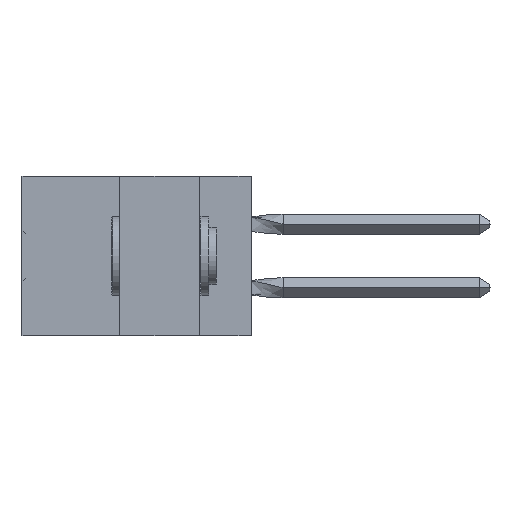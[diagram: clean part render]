
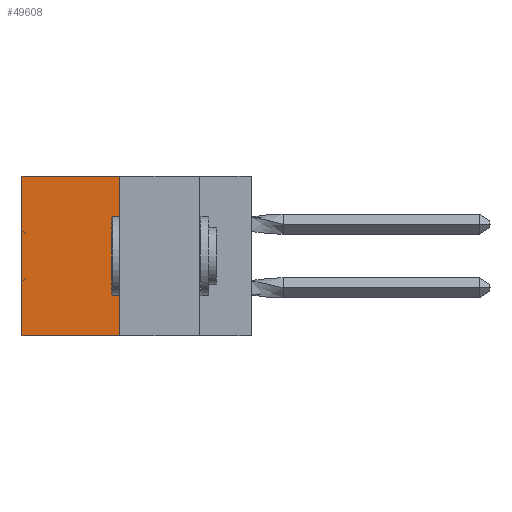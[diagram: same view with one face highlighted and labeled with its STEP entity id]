
A CAD part, left-side view. The second image highlights one B-rep face of the part: STEP entity #49608.
In plain terms, the highlighted planar face has unit normal (-1, 0, 0).
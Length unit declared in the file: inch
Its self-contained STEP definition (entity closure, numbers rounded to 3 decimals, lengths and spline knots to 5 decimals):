
#1169 = FACE_OUTER_BOUND ( 'NONE', #30408, .T. ) ;
#4736 = VECTOR ( 'NONE', #14009, 39.37008 ) ;
#5809 = VECTOR ( 'NONE', #36011, 39.37008 ) ;
#7497 = DIRECTION ( 'NONE',  ( 0., 1., 0. ) ) ;
#10159 = DIRECTION ( 'NONE',  ( 1., 0., 0. ) ) ;
#11826 = VERTEX_POINT ( 'NONE', #25598 ) ;
#12206 = LINE ( 'NONE', #53501, #4736 ) ;
#12739 = ORIENTED_EDGE ( 'NONE', *, *, #55975, .F. ) ;
#13294 = ORIENTED_EDGE ( 'NONE', *, *, #40919, .T. ) ;
#14009 = DIRECTION ( 'NONE',  ( 0., 0., -1. ) ) ;
#16894 = CARTESIAN_POINT ( 'NONE',  ( 0.305, 0.413, -0.5 ) ) ;
#19998 = EDGE_CURVE ( 'NONE', #11826, #40989, #12206, .T. ) ;
#22746 = CARTESIAN_POINT ( 'NONE',  ( 0.305, 0.413, -0.5 ) ) ;
#23274 = EDGE_CURVE ( 'NONE', #36505, #25533, #39822, .T. ) ;
#25533 = VERTEX_POINT ( 'NONE', #16894 ) ;
#25598 = CARTESIAN_POINT ( 'NONE',  ( 0.305, 0.72, 0. ) ) ;
#26746 = DIRECTION ( 'NONE',  ( 0., 1., 0. ) ) ;
#28204 = AXIS2_PLACEMENT_3D ( 'NONE', #22746, #10159, #40622 ) ;
#30408 = EDGE_LOOP ( 'NONE', ( #51049, #12739, #38060, #13294 ) ) ;
#31680 = VECTOR ( 'NONE', #7497, 39.37008 ) ;
#33910 = CARTESIAN_POINT ( 'NONE',  ( 0.305, 0.413, 0. ) ) ;
#34070 = VECTOR ( 'NONE', #26746, 39.37008 ) ;
#36011 = DIRECTION ( 'NONE',  ( 0., 0., -1. ) ) ;
#36232 = PLANE ( 'NONE',  #28204 ) ;
#36505 = VERTEX_POINT ( 'NONE', #37008 ) ;
#37008 = CARTESIAN_POINT ( 'NONE',  ( 0.305, 0.413, 0. ) ) ;
#38060 = ORIENTED_EDGE ( 'NONE', *, *, #23274, .F. ) ;
#39822 = LINE ( 'NONE', #44814, #5809 ) ;
#39830 = LINE ( 'NONE', #33910, #31680 ) ;
#39969 = CARTESIAN_POINT ( 'NONE',  ( 0.305, 0.72, -0.5 ) ) ;
#40622 = DIRECTION ( 'NONE',  ( 0., 0., -1. ) ) ;
#40919 = EDGE_CURVE ( 'NONE', #36505, #11826, #39830, .T. ) ;
#40989 = VERTEX_POINT ( 'NONE', #39969 ) ;
#43531 = CARTESIAN_POINT ( 'NONE',  ( 0.305, 0.413, -0.5 ) ) ;
#44814 = CARTESIAN_POINT ( 'NONE',  ( 0.305, 0.413, -0.5 ) ) ;
#49608 = ADVANCED_FACE ( 'NONE', ( #1169 ), #36232, .F. ) ;
#49937 = LINE ( 'NONE', #43531, #34070 ) ;
#51049 = ORIENTED_EDGE ( 'NONE', *, *, #19998, .T. ) ;
#53501 = CARTESIAN_POINT ( 'NONE',  ( 0.305, 0.72, -0.5 ) ) ;
#55975 = EDGE_CURVE ( 'NONE', #25533, #40989, #49937, .T. ) ;
